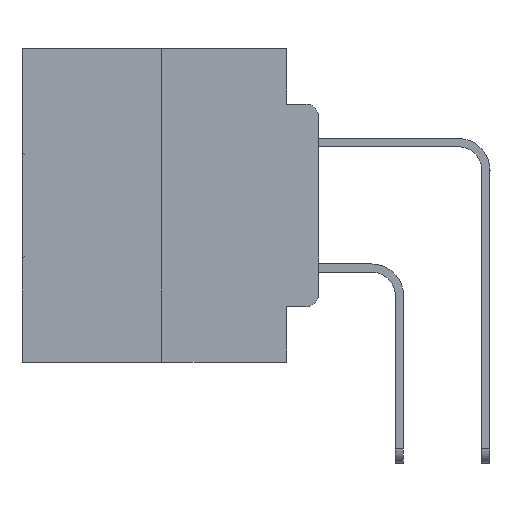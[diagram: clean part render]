
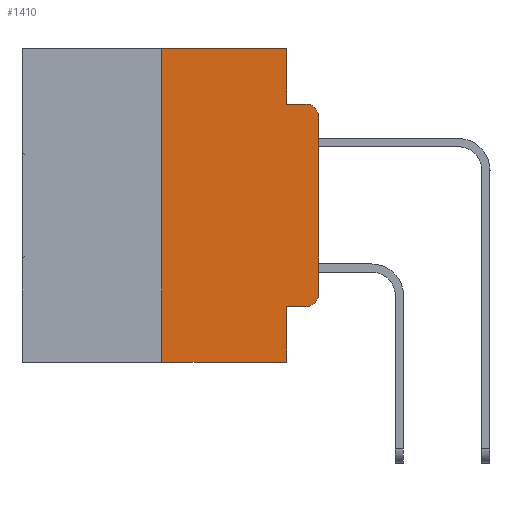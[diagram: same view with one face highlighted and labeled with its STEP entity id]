
A CAD part, left-side view. The second image highlights one B-rep face of the part: STEP entity #1410.
In plain terms, the highlighted planar face has unit normal (-1, 0, 0).
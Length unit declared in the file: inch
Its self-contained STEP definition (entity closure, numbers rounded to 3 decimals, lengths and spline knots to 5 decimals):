
#1301 = EDGE_CURVE ( 'NONE', #19515, #7419, #20807, .T. ) ;
#1410 = ADVANCED_FACE ( 'NONE', ( #9623 ), #17035, .F. ) ;
#1427 = DIRECTION ( 'NONE',  ( 0., -1., 0. ) ) ;
#1824 = ORIENTED_EDGE ( 'NONE', *, *, #26341, .T. ) ;
#2134 = DIRECTION ( 'NONE',  ( 0., -1., 0. ) ) ;
#2172 = LINE ( 'NONE', #29179, #24512 ) ;
#2370 = CARTESIAN_POINT ( 'NONE',  ( 0., 0.02, -0.1085 ) ) ;
#2569 = AXIS2_PLACEMENT_3D ( 'NONE', #21949, #17142, #4813 ) ;
#2814 = DIRECTION ( 'NONE',  ( 0., 0., -1. ) ) ;
#3181 = LINE ( 'NONE', #16041, #13188 ) ;
#3605 = ORIENTED_EDGE ( 'NONE', *, *, #9062, .T. ) ;
#3834 = AXIS2_PLACEMENT_3D ( 'NONE', #6179, #28477, #28169 ) ;
#3947 = DIRECTION ( 'NONE',  ( 0., 0., 1. ) ) ;
#4724 = DIRECTION ( 'NONE',  ( 0., 0., 1. ) ) ;
#4802 = VERTEX_POINT ( 'NONE', #16754 ) ;
#4813 = DIRECTION ( 'NONE',  ( 0., 0., -1. ) ) ;
#5132 = ORIENTED_EDGE ( 'NONE', *, *, #1301, .F. ) ;
#5179 = DIRECTION ( 'NONE',  ( 0., -1., 0. ) ) ;
#5225 = CARTESIAN_POINT ( 'NONE',  ( 0., 0.051, -0.5 ) ) ;
#5444 = ORIENTED_EDGE ( 'NONE', *, *, #17312, .T. ) ;
#5923 = CARTESIAN_POINT ( 'NONE',  ( 0., 0.051, -0.4115 ) ) ;
#6179 = CARTESIAN_POINT ( 'NONE',  ( 0., 0.02, -0.3915 ) ) ;
#6180 = LINE ( 'NONE', #23491, #25486 ) ;
#6234 = LINE ( 'NONE', #15104, #13612 ) ;
#6871 = VERTEX_POINT ( 'NONE', #13643 ) ;
#7232 = VERTEX_POINT ( 'NONE', #21469 ) ;
#7419 = VERTEX_POINT ( 'NONE', #29609 ) ;
#7741 = CARTESIAN_POINT ( 'NONE',  ( 0., 0.02, -0.4115 ) ) ;
#7800 = VECTOR ( 'NONE', #12502, 39.37008 ) ;
#8342 = ORIENTED_EDGE ( 'NONE', *, *, #10910, .T. ) ;
#9062 = EDGE_CURVE ( 'NONE', #4802, #30693, #17108, .T. ) ;
#9623 = FACE_OUTER_BOUND ( 'NONE', #19051, .T. ) ;
#10910 = EDGE_CURVE ( 'NONE', #28606, #7232, #13159, .T. ) ;
#11801 = VECTOR ( 'NONE', #30598, 39.37008 ) ;
#12176 = ORIENTED_EDGE ( 'NONE', *, *, #17068, .F. ) ;
#12197 = CARTESIAN_POINT ( 'NONE',  ( 0., 0.051, -0.0885 ) ) ;
#12502 = DIRECTION ( 'NONE',  ( 0., -1., 0. ) ) ;
#13159 = CIRCLE ( 'NONE', #25337, 0.02 ) ;
#13188 = VECTOR ( 'NONE', #3947, 39.37008 ) ;
#13612 = VECTOR ( 'NONE', #2814, 39.37008 ) ;
#13643 = CARTESIAN_POINT ( 'NONE',  ( 0., 0., -0.3915 ) ) ;
#14287 = ORIENTED_EDGE ( 'NONE', *, *, #22209, .T. ) ;
#15026 = VECTOR ( 'NONE', #2134, 39.37008 ) ;
#15104 = CARTESIAN_POINT ( 'NONE',  ( 0., 0.051, 0. ) ) ;
#15283 = LINE ( 'NONE', #30049, #11801 ) ;
#15746 = EDGE_CURVE ( 'NONE', #30192, #30693, #6234, .T. ) ;
#16041 = CARTESIAN_POINT ( 'NONE',  ( 0., 0.25, 0. ) ) ;
#16754 = CARTESIAN_POINT ( 'NONE',  ( 0., 0.25, -0.5 ) ) ;
#17035 = PLANE ( 'NONE',  #2569 ) ;
#17068 = EDGE_CURVE ( 'NONE', #22177, #7232, #27408, .T. ) ;
#17108 = LINE ( 'NONE', #29419, #7800 ) ;
#17142 = DIRECTION ( 'NONE',  ( 1., 0., 0. ) ) ;
#17312 = EDGE_CURVE ( 'NONE', #30192, #19648, #6180, .T. ) ;
#17580 = DIRECTION ( 'NONE',  ( -1., 0., 0. ) ) ;
#19051 = EDGE_LOOP ( 'NONE', ( #14287, #8342, #12176, #29891, #5132, #29563, #3605, #28386, #5444, #1824 ) ) ;
#19515 = VERTEX_POINT ( 'NONE', #31357 ) ;
#19648 = VERTEX_POINT ( 'NONE', #7741 ) ;
#19871 = EDGE_CURVE ( 'NONE', #7419, #22177, #15283, .T. ) ;
#20807 = LINE ( 'NONE', #31428, #15026 ) ;
#21469 = CARTESIAN_POINT ( 'NONE',  ( 0., 0.02, -0.0885 ) ) ;
#21653 = VECTOR ( 'NONE', #5179, 39.37008 ) ;
#21949 = CARTESIAN_POINT ( 'NONE',  ( 0., 0.473, 0. ) ) ;
#22177 = VERTEX_POINT ( 'NONE', #31448 ) ;
#22209 = EDGE_CURVE ( 'NONE', #6871, #28606, #2172, .T. ) ;
#23491 = CARTESIAN_POINT ( 'NONE',  ( 0., 0.051, -0.4115 ) ) ;
#24512 = VECTOR ( 'NONE', #4724, 39.37008 ) ;
#24572 = EDGE_CURVE ( 'NONE', #4802, #19515, #3181, .T. ) ;
#25337 = AXIS2_PLACEMENT_3D ( 'NONE', #2370, #17580, #29603 ) ;
#25486 = VECTOR ( 'NONE', #1427, 39.37008 ) ;
#26341 = EDGE_CURVE ( 'NONE', #19648, #6871, #28127, .T. ) ;
#26814 = CARTESIAN_POINT ( 'NONE',  ( 0., 0., -0.1085 ) ) ;
#27408 = LINE ( 'NONE', #12197, #21653 ) ;
#28127 = CIRCLE ( 'NONE', #3834, 0.02 ) ;
#28169 = DIRECTION ( 'NONE',  ( 0., 0., -1. ) ) ;
#28386 = ORIENTED_EDGE ( 'NONE', *, *, #15746, .F. ) ;
#28477 = DIRECTION ( 'NONE',  ( -1., 0., 0. ) ) ;
#28606 = VERTEX_POINT ( 'NONE', #26814 ) ;
#29179 = CARTESIAN_POINT ( 'NONE',  ( 0., 0., 0. ) ) ;
#29419 = CARTESIAN_POINT ( 'NONE',  ( 0., 0.473, -0.5 ) ) ;
#29563 = ORIENTED_EDGE ( 'NONE', *, *, #24572, .F. ) ;
#29603 = DIRECTION ( 'NONE',  ( 0., 0., -1. ) ) ;
#29609 = CARTESIAN_POINT ( 'NONE',  ( 0., 0.051, 0. ) ) ;
#29891 = ORIENTED_EDGE ( 'NONE', *, *, #19871, .F. ) ;
#30049 = CARTESIAN_POINT ( 'NONE',  ( 0., 0.051, 0. ) ) ;
#30192 = VERTEX_POINT ( 'NONE', #5923 ) ;
#30598 = DIRECTION ( 'NONE',  ( 0., 0., -1. ) ) ;
#30693 = VERTEX_POINT ( 'NONE', #5225 ) ;
#31357 = CARTESIAN_POINT ( 'NONE',  ( 0., 0.25, 0. ) ) ;
#31428 = CARTESIAN_POINT ( 'NONE',  ( 0., 0.473, 0. ) ) ;
#31448 = CARTESIAN_POINT ( 'NONE',  ( 0., 0.051, -0.0885 ) ) ;
